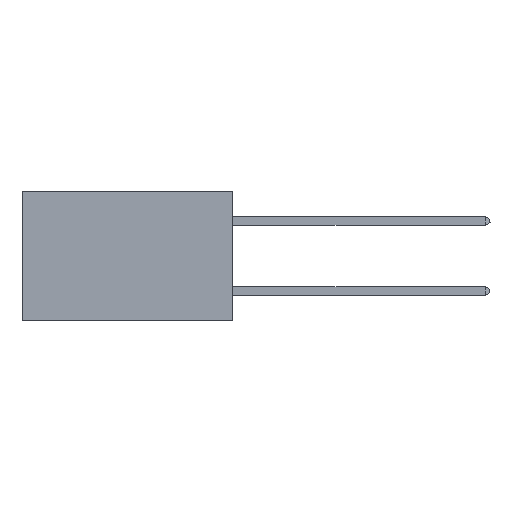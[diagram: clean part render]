
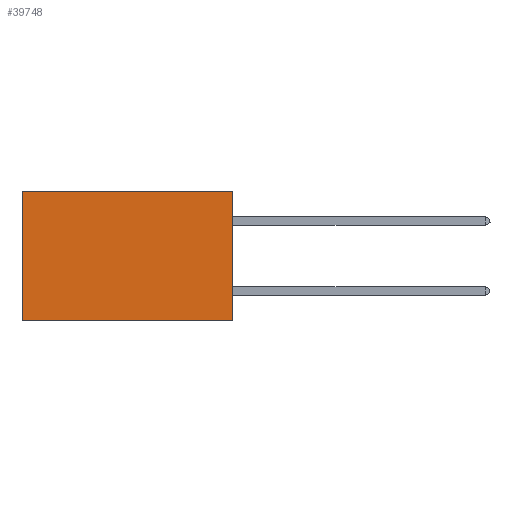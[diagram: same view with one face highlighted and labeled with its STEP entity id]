
A CAD part, left-side view. The second image highlights one B-rep face of the part: STEP entity #39748.
In plain terms, the highlighted planar face has unit normal (-1, 0, 0).
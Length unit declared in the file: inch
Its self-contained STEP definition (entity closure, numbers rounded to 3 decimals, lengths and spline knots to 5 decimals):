
#4444 = ORIENTED_EDGE ( 'NONE', *, *, #29908, .T. ) ;
#5135 = ORIENTED_EDGE ( 'NONE', *, *, #31662, .F. ) ;
#5547 = ORIENTED_EDGE ( 'NONE', *, *, #23667, .F. ) ;
#5887 = VECTOR ( 'NONE', #33271, 39.37008 ) ;
#6673 = DIRECTION ( 'NONE',  ( 0., 0., -1. ) ) ;
#6693 = CARTESIAN_POINT ( 'NONE',  ( 0.2875, 0., 0. ) ) ;
#7231 = DIRECTION ( 'NONE',  ( 0., 0., -1. ) ) ;
#7384 = VERTEX_POINT ( 'NONE', #11418 ) ;
#8269 = CARTESIAN_POINT ( 'NONE',  ( 0.2875, 0., 0. ) ) ;
#9943 = CARTESIAN_POINT ( 'NONE',  ( 0.2875, 0., 0. ) ) ;
#11418 = CARTESIAN_POINT ( 'NONE',  ( 0.2875, 0.6, 0. ) ) ;
#13178 = VERTEX_POINT ( 'NONE', #26388 ) ;
#14939 = EDGE_LOOP ( 'NONE', ( #4444, #5547, #5135, #32029 ) ) ;
#15040 = CARTESIAN_POINT ( 'NONE',  ( 0.2875, 0.6, -0.37 ) ) ;
#18008 = AXIS2_PLACEMENT_3D ( 'NONE', #8269, #40751, #21559 ) ;
#18290 = PLANE ( 'NONE',  #18008 ) ;
#18295 = LINE ( 'NONE', #26361, #27909 ) ;
#19490 = LINE ( 'NONE', #33265, #35620 ) ;
#21559 = DIRECTION ( 'NONE',  ( 0., 0., -1. ) ) ;
#23667 = EDGE_CURVE ( 'NONE', #13178, #37554, #24427, .T. ) ;
#24427 = LINE ( 'NONE', #36475, #5887 ) ;
#24715 = EDGE_CURVE ( 'NONE', #41602, #7384, #34429, .T. ) ;
#26361 = CARTESIAN_POINT ( 'NONE',  ( 0.2875, 0., 0. ) ) ;
#26388 = CARTESIAN_POINT ( 'NONE',  ( 0.2875, 0., -0.37 ) ) ;
#27909 = VECTOR ( 'NONE', #6673, 39.37008 ) ;
#28903 = FACE_OUTER_BOUND ( 'NONE', #14939, .T. ) ;
#29908 = EDGE_CURVE ( 'NONE', #7384, #37554, #19490, .T. ) ;
#31662 = EDGE_CURVE ( 'NONE', #41602, #13178, #18295, .T. ) ;
#32029 = ORIENTED_EDGE ( 'NONE', *, *, #24715, .T. ) ;
#32805 = DIRECTION ( 'NONE',  ( 0., 1., 0. ) ) ;
#33265 = CARTESIAN_POINT ( 'NONE',  ( 0.2875, 0.6, 0. ) ) ;
#33271 = DIRECTION ( 'NONE',  ( 0., 1., 0. ) ) ;
#33431 = VECTOR ( 'NONE', #32805, 39.37008 ) ;
#34429 = LINE ( 'NONE', #9943, #33431 ) ;
#35620 = VECTOR ( 'NONE', #7231, 39.37008 ) ;
#36475 = CARTESIAN_POINT ( 'NONE',  ( 0.2875, 0., -0.37 ) ) ;
#37554 = VERTEX_POINT ( 'NONE', #15040 ) ;
#39748 = ADVANCED_FACE ( 'NONE', ( #28903 ), #18290, .F. ) ;
#40751 = DIRECTION ( 'NONE',  ( 1., 0., 0. ) ) ;
#41602 = VERTEX_POINT ( 'NONE', #6693 ) ;
